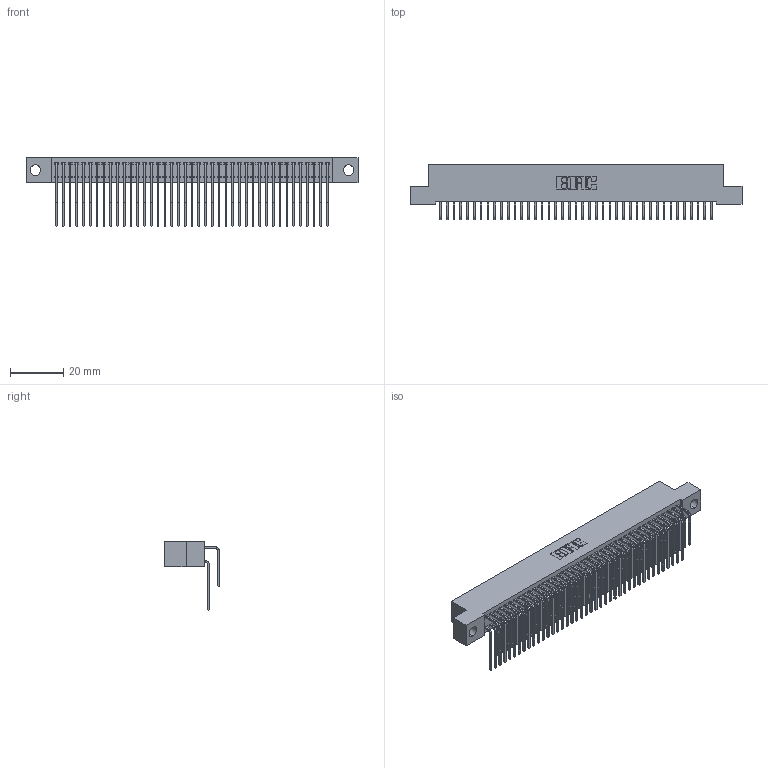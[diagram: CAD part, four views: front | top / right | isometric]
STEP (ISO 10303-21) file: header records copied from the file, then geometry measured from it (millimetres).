
FILE_DESCRIPTION (( 'STEP AP203' ), '1' );
FILE_NAME ('392-082-559-204.STEP', '2018-08-18T04:04:55', ( '' ), ( '' ), 'SwSTEP 2.0', 'SolidWorks 2016', '' );
FILE_SCHEMA (( 'CONFIG_CONTROL_DESIGN' ));
Length unit declared in the file: inch
Products named in the file (4): 392-082-559-204; 342 Part_.156 TH; 345-292-001_558 559 Tail - 1; 345-292-001_559 Tail - 2
Assembly tree (83 placements, depth 2):
  392-082-559-204
    342 Part_.156 TH
    345-292-001_558 559 Tail - 1  x41
    345-292-001_559 Tail - 2  x41
Bounding box: 124.46 x 20.64 x 25.78 mm (x, y, z)
Volume: 11564 mm3; surface area: 20762.7 mm2
Topology: 83 solids, 83 shells, 4538 faces, 13501 edges, 8890 vertices
Faces by surface type: plane 3182, cylinder 1356
Entity records: 28161 total; most frequent: CARTESIAN_POINT 4717, ORIENTED_EDGE 4602, DIRECTION 4013, EDGE_CURVE 2301, VECTOR 2133, LINE 2133, VERTEX_POINT 1530, AXIS2_PLACEMENT_3D 940
